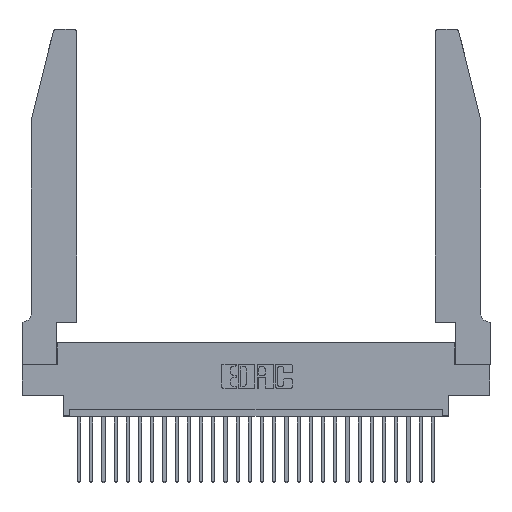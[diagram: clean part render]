
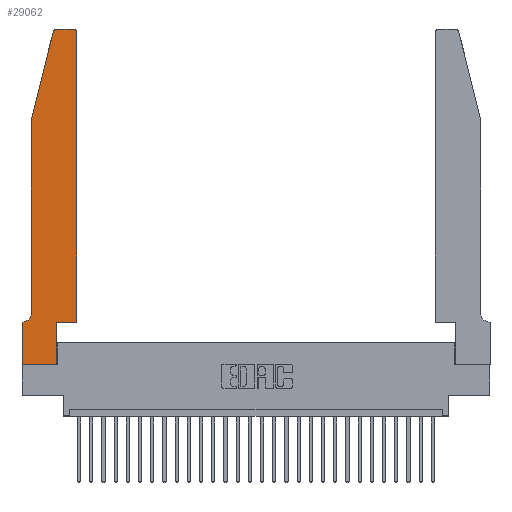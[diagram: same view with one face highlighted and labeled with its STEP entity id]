
A CAD part, top view. The second image highlights one B-rep face of the part: STEP entity #29062.
In plain terms, the highlighted planar face has unit normal (0, 0, 1).
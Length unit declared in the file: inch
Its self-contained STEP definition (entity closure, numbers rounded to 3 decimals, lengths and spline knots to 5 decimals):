
#39 = CARTESIAN_POINT ( 'NONE',  ( 0.2865, 0., 0.37 ) ) ;
#66 = VERTEX_POINT ( 'NONE', #39 ) ;
#277 = AXIS2_PLACEMENT_3D ( 'NONE', #5104, #16141, #23221 ) ;
#545 = VERTEX_POINT ( 'NONE', #23178 ) ;
#1252 = CARTESIAN_POINT ( 'NONE',  ( 0.2865, 0.35, 0.37 ) ) ;
#1710 = ORIENTED_EDGE ( 'NONE', *, *, #17701, .T. ) ;
#2060 = CARTESIAN_POINT ( 'NONE',  ( 0., 0., 0.37 ) ) ;
#2197 = ORIENTED_EDGE ( 'NONE', *, *, #27397, .T. ) ;
#2732 = ORIENTED_EDGE ( 'NONE', *, *, #3437, .T. ) ;
#3129 = VERTEX_POINT ( 'NONE', #21649 ) ;
#3437 = EDGE_CURVE ( 'NONE', #28608, #25257, #14887, .T. ) ;
#3595 = CARTESIAN_POINT ( 'NONE',  ( 0.0755, 2., 0.37 ) ) ;
#3832 = ORIENTED_EDGE ( 'NONE', *, *, #23303, .T. ) ;
#4111 = LINE ( 'NONE', #1252, #16072 ) ;
#5104 = CARTESIAN_POINT ( 'NONE',  ( 0., 0.35, 0.37 ) ) ;
#5183 = VERTEX_POINT ( 'NONE', #13900 ) ;
#5486 = VECTOR ( 'NONE', #17675, 39.37008 ) ;
#5519 = DIRECTION ( 'NONE',  ( 1., 0., 0. ) ) ;
#5631 = CARTESIAN_POINT ( 'NONE',  ( 0.0055, 0.35, 0.37 ) ) ;
#5840 = LINE ( 'NONE', #26545, #5486 ) ;
#6127 = VECTOR ( 'NONE', #8106, 39.37008 ) ;
#6672 = CARTESIAN_POINT ( 'NONE',  ( 0.2865, 0.35, 0.37 ) ) ;
#6948 = VERTEX_POINT ( 'NONE', #11062 ) ;
#7225 = VECTOR ( 'NONE', #18259, 39.37008 ) ;
#7329 = EDGE_CURVE ( 'NONE', #3129, #6948, #21049, .T. ) ;
#7973 = ORIENTED_EDGE ( 'NONE', *, *, #19298, .T. ) ;
#7988 = VECTOR ( 'NONE', #5519, 39.37008 ) ;
#8106 = DIRECTION ( 'NONE',  ( -1., 0., 0. ) ) ;
#8337 = EDGE_CURVE ( 'NONE', #22570, #28608, #15682, .T. ) ;
#8528 = VERTEX_POINT ( 'NONE', #17049 ) ;
#8632 = DIRECTION ( 'NONE',  ( 0., 0., 1. ) ) ;
#8926 = DIRECTION ( 'NONE',  ( 1., 0., 0. ) ) ;
#9752 = DIRECTION ( 'NONE',  ( 0., 0., -1. ) ) ;
#9954 = CARTESIAN_POINT ( 'NONE',  ( 0.25487, 2.72718, 0.37 ) ) ;
#10826 = LINE ( 'NONE', #2060, #15060 ) ;
#11057 = LINE ( 'NONE', #19346, #6127 ) ;
#11062 = CARTESIAN_POINT ( 'NONE',  ( 0.4505, 2.72, 0.37 ) ) ;
#11512 = CARTESIAN_POINT ( 'NONE',  ( 0.0055, 0.42, 0.37 ) ) ;
#11739 = CARTESIAN_POINT ( 'NONE',  ( 0.2605, 2.75, 0.37 ) ) ;
#12306 = EDGE_LOOP ( 'NONE', ( #26286, #14743, #16984, #2732, #18313, #3832, #25696, #26180, #1710, #7973, #13250, #2197 ) ) ;
#12312 = CARTESIAN_POINT ( 'NONE',  ( 0.0755, 0.42, 0.37 ) ) ;
#12699 = EDGE_CURVE ( 'NONE', #5183, #22570, #27252, .T. ) ;
#13250 = ORIENTED_EDGE ( 'NONE', *, *, #7329, .T. ) ;
#13323 = VERTEX_POINT ( 'NONE', #5631 ) ;
#13630 = DIRECTION ( 'NONE',  ( 0., 0., 1. ) ) ;
#13900 = CARTESIAN_POINT ( 'NONE',  ( 0.284, 2.75, 0.37 ) ) ;
#14044 = DIRECTION ( 'NONE',  ( 0., -1., 0. ) ) ;
#14344 = DIRECTION ( 'NONE',  ( -1., 0., 0. ) ) ;
#14743 = ORIENTED_EDGE ( 'NONE', *, *, #12699, .T. ) ;
#14887 = LINE ( 'NONE', #18316, #24062 ) ;
#15037 = VECTOR ( 'NONE', #21900, 39.37008 ) ;
#15060 = VECTOR ( 'NONE', #17778, 39.37008 ) ;
#15290 = FACE_OUTER_BOUND ( 'NONE', #12306, .T. ) ;
#15682 = LINE ( 'NONE', #3595, #22713 ) ;
#16072 = VECTOR ( 'NONE', #23464, 39.37008 ) ;
#16141 = DIRECTION ( 'NONE',  ( 0., 0., 1. ) ) ;
#16337 = PLANE ( 'NONE',  #277 ) ;
#16355 = AXIS2_PLACEMENT_3D ( 'NONE', #24315, #8632, #8926 ) ;
#16764 = CARTESIAN_POINT ( 'NONE',  ( 0.4505, 0.35, 0.37 ) ) ;
#16984 = ORIENTED_EDGE ( 'NONE', *, *, #8337, .T. ) ;
#17049 = CARTESIAN_POINT ( 'NONE',  ( 0.4205, 2.75, 0.37 ) ) ;
#17287 = AXIS2_PLACEMENT_3D ( 'NONE', #11512, #9752, #14344 ) ;
#17675 = DIRECTION ( 'NONE',  ( 1., 0., 0. ) ) ;
#17701 = EDGE_CURVE ( 'NONE', #66, #23185, #4111, .T. ) ;
#17778 = DIRECTION ( 'NONE',  ( 0., -1., 0. ) ) ;
#17968 = AXIS2_PLACEMENT_3D ( 'NONE', #20470, #13630, #20668 ) ;
#18142 = CARTESIAN_POINT ( 'NONE',  ( 0., 0.35, 0.37 ) ) ;
#18259 = DIRECTION ( 'NONE',  ( -1., 0., 0. ) ) ;
#18313 = ORIENTED_EDGE ( 'NONE', *, *, #19204, .T. ) ;
#18316 = CARTESIAN_POINT ( 'NONE',  ( 0.0755, 2., 0.37 ) ) ;
#19204 = EDGE_CURVE ( 'NONE', #25257, #13323, #25243, .T. ) ;
#19291 = LINE ( 'NONE', #16764, #7988 ) ;
#19298 = EDGE_CURVE ( 'NONE', #23185, #3129, #19291, .T. ) ;
#19346 = CARTESIAN_POINT ( 'NONE',  ( 0.0755, 0.35, 0.37 ) ) ;
#19952 = LINE ( 'NONE', #11739, #7225 ) ;
#20470 = CARTESIAN_POINT ( 'NONE',  ( 0.4205, 2.72, 0.37 ) ) ;
#20668 = DIRECTION ( 'NONE',  ( 1., 0., 0. ) ) ;
#21049 = LINE ( 'NONE', #28724, #15037 ) ;
#21394 = CIRCLE ( 'NONE', #17968, 0.03 ) ;
#21649 = CARTESIAN_POINT ( 'NONE',  ( 0.4505, 0.35, 0.37 ) ) ;
#21900 = DIRECTION ( 'NONE',  ( 0., 1., 0. ) ) ;
#22156 = EDGE_CURVE ( 'NONE', #545, #66, #5840, .T. ) ;
#22570 = VERTEX_POINT ( 'NONE', #9954 ) ;
#22713 = VECTOR ( 'NONE', #26152, 39.37008 ) ;
#23178 = CARTESIAN_POINT ( 'NONE',  ( 0., 0., 0.37 ) ) ;
#23185 = VERTEX_POINT ( 'NONE', #6672 ) ;
#23221 = DIRECTION ( 'NONE',  ( 1., 0., 0. ) ) ;
#23303 = EDGE_CURVE ( 'NONE', #13323, #25042, #11057, .T. ) ;
#23464 = DIRECTION ( 'NONE',  ( 0., 1., 0. ) ) ;
#24062 = VECTOR ( 'NONE', #14044, 39.37008 ) ;
#24315 = CARTESIAN_POINT ( 'NONE',  ( 0.284, 2.72, 0.37 ) ) ;
#25042 = VERTEX_POINT ( 'NONE', #18142 ) ;
#25243 = CIRCLE ( 'NONE', #17287, 0.07 ) ;
#25257 = VERTEX_POINT ( 'NONE', #12312 ) ;
#25696 = ORIENTED_EDGE ( 'NONE', *, *, #26707, .T. ) ;
#26152 = DIRECTION ( 'NONE',  ( -0.239, -0.971, 0. ) ) ;
#26180 = ORIENTED_EDGE ( 'NONE', *, *, #22156, .T. ) ;
#26286 = ORIENTED_EDGE ( 'NONE', *, *, #28301, .T. ) ;
#26347 = CARTESIAN_POINT ( 'NONE',  ( 0.0755, 2., 0.37 ) ) ;
#26545 = CARTESIAN_POINT ( 'NONE',  ( 0., 0., 0.37 ) ) ;
#26707 = EDGE_CURVE ( 'NONE', #25042, #545, #10826, .T. ) ;
#27252 = CIRCLE ( 'NONE', #16355, 0.03 ) ;
#27397 = EDGE_CURVE ( 'NONE', #6948, #8528, #21394, .T. ) ;
#28301 = EDGE_CURVE ( 'NONE', #8528, #5183, #19952, .T. ) ;
#28608 = VERTEX_POINT ( 'NONE', #26347 ) ;
#28724 = CARTESIAN_POINT ( 'NONE',  ( 0.4505, 0.35, 0.37 ) ) ;
#29062 = ADVANCED_FACE ( 'NONE', ( #15290 ), #16337, .T. ) ;
